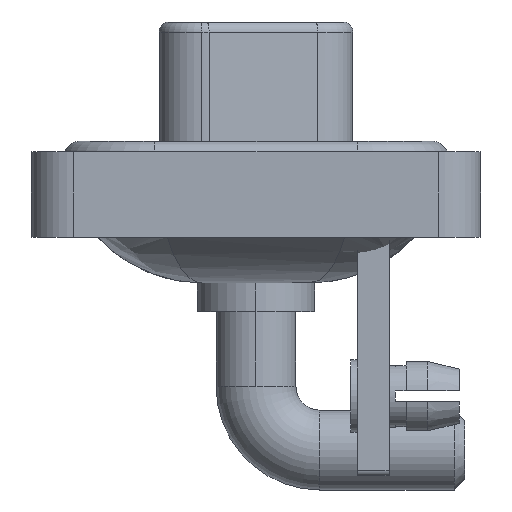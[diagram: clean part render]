
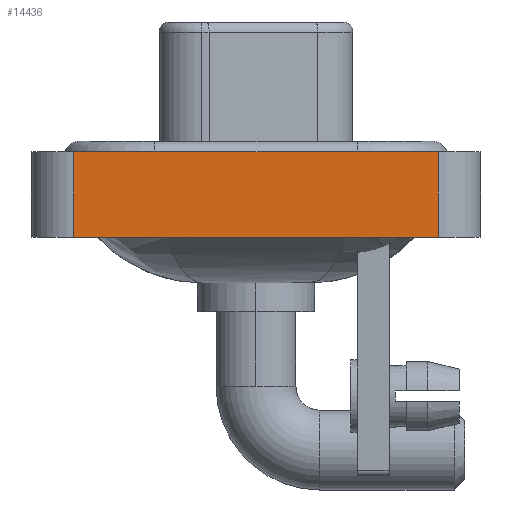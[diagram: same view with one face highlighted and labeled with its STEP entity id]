
A CAD part, left-side view. The second image highlights one B-rep face of the part: STEP entity #14436.
In plain terms, the highlighted planar face has unit normal (-1, 0, 0).
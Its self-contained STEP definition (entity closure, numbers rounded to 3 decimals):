
#491 = DIRECTION ( 'NONE',  ( -1., 0., 0. ) ) ;
#525 = EDGE_CURVE ( 'NONE', #20440, #1779, #11957, .T. ) ;
#778 = DIRECTION ( 'NONE',  ( 0., -1., 0. ) ) ;
#1158 = AXIS2_PLACEMENT_3D ( 'NONE', #10142, #491, #13132 ) ;
#1779 = VERTEX_POINT ( 'NONE', #14768 ) ;
#1958 = ORIENTED_EDGE ( 'NONE', *, *, #525, .T. ) ;
#3245 = ORIENTED_EDGE ( 'NONE', *, *, #4141, .F. ) ;
#3819 = EDGE_CURVE ( 'NONE', #13690, #13689, #10722, .T. ) ;
#4141 = EDGE_CURVE ( 'NONE', #13689, #1779, #12687, .T. ) ;
#4809 = DIRECTION ( 'NONE',  ( 0., -1., 0. ) ) ;
#4921 = CARTESIAN_POINT ( 'NONE',  ( -7.35, 8.55, 0.4 ) ) ;
#5507 = EDGE_CURVE ( 'NONE', #13690, #20440, #8448, .T. ) ;
#8448 = LINE ( 'NONE', #14757, #16041 ) ;
#10142 = CARTESIAN_POINT ( 'NONE',  ( -7.35, -8.55, -3.6 ) ) ;
#10196 = VECTOR ( 'NONE', #13818, 1000. ) ;
#10722 = LINE ( 'NONE', #15473, #19998 ) ;
#11588 = ORIENTED_EDGE ( 'NONE', *, *, #3819, .F. ) ;
#11957 = LINE ( 'NONE', #18354, #10196 ) ;
#12445 = VECTOR ( 'NONE', #4809, 1000. ) ;
#12509 = CARTESIAN_POINT ( 'NONE',  ( -7.35, 8.55, -3.6 ) ) ;
#12687 = LINE ( 'NONE', #18988, #12445 ) ;
#13035 = FACE_OUTER_BOUND ( 'NONE', #18899, .T. ) ;
#13132 = DIRECTION ( 'NONE',  ( 0., 0., 1. ) ) ;
#13461 = PLANE ( 'NONE',  #1158 ) ;
#13689 = VERTEX_POINT ( 'NONE', #4921 ) ;
#13690 = VERTEX_POINT ( 'NONE', #12509 ) ;
#13818 = DIRECTION ( 'NONE',  ( 0., 0., 1. ) ) ;
#14436 = ADVANCED_FACE ( 'NONE', ( #13035 ), #13461, .T. ) ;
#14677 = CARTESIAN_POINT ( 'NONE',  ( -7.35, -8.55, -3.6 ) ) ;
#14757 = CARTESIAN_POINT ( 'NONE',  ( -7.35, -8.55, -3.6 ) ) ;
#14768 = CARTESIAN_POINT ( 'NONE',  ( -7.35, -8.55, 0.4 ) ) ;
#15473 = CARTESIAN_POINT ( 'NONE',  ( -7.35, 8.55, -3.6 ) ) ;
#15936 = ORIENTED_EDGE ( 'NONE', *, *, #5507, .T. ) ;
#16041 = VECTOR ( 'NONE', #778, 1000. ) ;
#17013 = DIRECTION ( 'NONE',  ( 0., 0., 1. ) ) ;
#18354 = CARTESIAN_POINT ( 'NONE',  ( -7.35, -8.55, -3.6 ) ) ;
#18899 = EDGE_LOOP ( 'NONE', ( #1958, #3245, #11588, #15936 ) ) ;
#18988 = CARTESIAN_POINT ( 'NONE',  ( -7.35, -8.55, 0.4 ) ) ;
#19998 = VECTOR ( 'NONE', #17013, 1000. ) ;
#20440 = VERTEX_POINT ( 'NONE', #14677 ) ;
